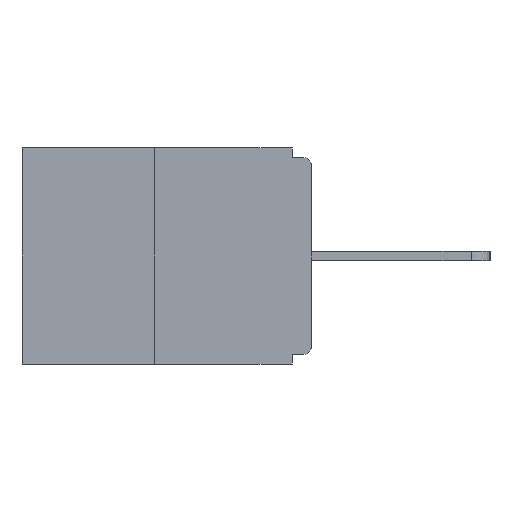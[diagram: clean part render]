
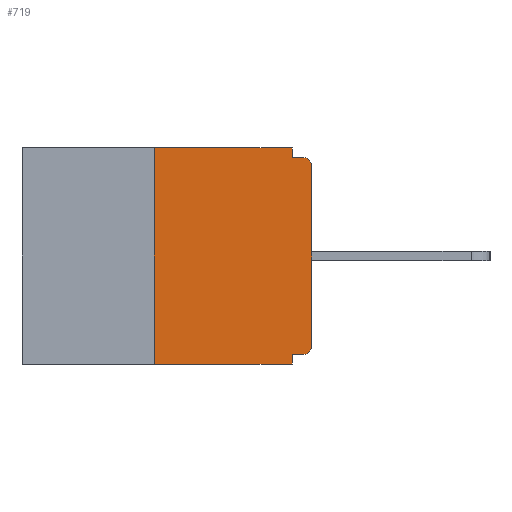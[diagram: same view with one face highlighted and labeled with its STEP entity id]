
A CAD part, left-side view. The second image highlights one B-rep face of the part: STEP entity #719.
In plain terms, the highlighted planar face has unit normal (-1, 0, 0).
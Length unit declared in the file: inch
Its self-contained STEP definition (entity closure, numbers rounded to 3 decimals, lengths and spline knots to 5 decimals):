
#126 = DIRECTION ( 'NONE',  ( 0., -1., 0. ) ) ;
#239 = DIRECTION ( 'NONE',  ( 0., 0., 1. ) ) ;
#290 = DIRECTION ( 'NONE',  ( 0., -1., 0. ) ) ;
#591 = VECTOR ( 'NONE', #10116, 39.37008 ) ;
#592 = VECTOR ( 'NONE', #1793, 39.37008 ) ;
#637 = EDGE_CURVE ( 'NONE', #10291, #11507, #8738, .T. ) ;
#719 = ADVANCED_FACE ( 'NONE', ( #7447 ), #3666, .F. ) ;
#789 = ORIENTED_EDGE ( 'NONE', *, *, #4757, .F. ) ;
#863 = LINE ( 'NONE', #10939, #592 ) ;
#873 = CARTESIAN_POINT ( 'NONE',  ( 0., 0.25, 0. ) ) ;
#1704 = CARTESIAN_POINT ( 'NONE',  ( 0., 0.46, 0. ) ) ;
#1740 = DIRECTION ( 'NONE',  ( -1., 0., 0. ) ) ;
#1793 = DIRECTION ( 'NONE',  ( 0., 0., 1. ) ) ;
#1847 = LINE ( 'NONE', #11578, #3069 ) ;
#1910 = CIRCLE ( 'NONE', #5224, 0.015 ) ;
#2091 = VERTEX_POINT ( 'NONE', #6015 ) ;
#2169 = DIRECTION ( 'NONE',  ( 0., 0., -1. ) ) ;
#2227 = DIRECTION ( 'NONE',  ( -1., 0., 0. ) ) ;
#2331 = ORIENTED_EDGE ( 'NONE', *, *, #2547, .T. ) ;
#2342 = EDGE_CURVE ( 'NONE', #5936, #8903, #7374, .T. ) ;
#2483 = ORIENTED_EDGE ( 'NONE', *, *, #2775, .T. ) ;
#2547 = EDGE_CURVE ( 'NONE', #4592, #10291, #863, .T. ) ;
#2624 = CARTESIAN_POINT ( 'NONE',  ( 0., 0.46, 0. ) ) ;
#2694 = VERTEX_POINT ( 'NONE', #5092 ) ;
#2775 = EDGE_CURVE ( 'NONE', #8818, #2091, #6390, .T. ) ;
#2864 = VECTOR ( 'NONE', #290, 39.37008 ) ;
#3030 = LINE ( 'NONE', #4143, #8489 ) ;
#3069 = VECTOR ( 'NONE', #12545, 39.37008 ) ;
#3420 = EDGE_CURVE ( 'NONE', #8818, #4256, #3030, .T. ) ;
#3666 = PLANE ( 'NONE',  #6430 ) ;
#4143 = CARTESIAN_POINT ( 'NONE',  ( 0., 0.25, 0. ) ) ;
#4256 = VERTEX_POINT ( 'NONE', #873 ) ;
#4377 = DIRECTION ( 'NONE',  ( 0., 1., 0. ) ) ;
#4575 = EDGE_CURVE ( 'NONE', #8903, #2091, #1847, .T. ) ;
#4592 = VERTEX_POINT ( 'NONE', #5552 ) ;
#4757 = EDGE_CURVE ( 'NONE', #2694, #11507, #11954, .T. ) ;
#5068 = EDGE_LOOP ( 'NONE', ( #11015, #7765, #2483, #12717, #10678, #7338, #2331, #10615, #789, #6046 ) ) ;
#5092 = CARTESIAN_POINT ( 'NONE',  ( 0., 0.031, -0.015 ) ) ;
#5144 = CARTESIAN_POINT ( 'NONE',  ( 0., 0., -0.015 ) ) ;
#5224 = AXIS2_PLACEMENT_3D ( 'NONE', #12027, #2227, #2169 ) ;
#5390 = CARTESIAN_POINT ( 'NONE',  ( 0., 0.031, 0. ) ) ;
#5540 = EDGE_CURVE ( 'NONE', #5936, #4592, #1910, .T. ) ;
#5552 = CARTESIAN_POINT ( 'NONE',  ( 0., 0., -0.313 ) ) ;
#5571 = DIRECTION ( 'NONE',  ( 0., 0., -1. ) ) ;
#5632 = DIRECTION ( 'NONE',  ( 0., 0., -1. ) ) ;
#5936 = VERTEX_POINT ( 'NONE', #6125 ) ;
#6015 = CARTESIAN_POINT ( 'NONE',  ( 0., 0.031, -0.343 ) ) ;
#6046 = ORIENTED_EDGE ( 'NONE', *, *, #6578, .F. ) ;
#6125 = CARTESIAN_POINT ( 'NONE',  ( 0., 0.015, -0.328 ) ) ;
#6169 = CARTESIAN_POINT ( 'NONE',  ( 0., 0.031, -0.328 ) ) ;
#6390 = LINE ( 'NONE', #8430, #2864 ) ;
#6430 = AXIS2_PLACEMENT_3D ( 'NONE', #2624, #10444, #5632 ) ;
#6578 = EDGE_CURVE ( 'NONE', #9125, #2694, #9363, .T. ) ;
#6613 = DIRECTION ( 'NONE',  ( 0., -1., 0. ) ) ;
#7257 = AXIS2_PLACEMENT_3D ( 'NONE', #12316, #1740, #5571 ) ;
#7297 = EDGE_CURVE ( 'NONE', #4256, #9125, #11570, .T. ) ;
#7338 = ORIENTED_EDGE ( 'NONE', *, *, #5540, .T. ) ;
#7374 = LINE ( 'NONE', #8422, #12171 ) ;
#7422 = CARTESIAN_POINT ( 'NONE',  ( 0., 0.015, -0.015 ) ) ;
#7447 = FACE_OUTER_BOUND ( 'NONE', #5068, .T. ) ;
#7634 = VECTOR ( 'NONE', #126, 39.37008 ) ;
#7658 = CARTESIAN_POINT ( 'NONE',  ( 0., 0., -0.03 ) ) ;
#7765 = ORIENTED_EDGE ( 'NONE', *, *, #3420, .F. ) ;
#8422 = CARTESIAN_POINT ( 'NONE',  ( 0., 0., -0.328 ) ) ;
#8430 = CARTESIAN_POINT ( 'NONE',  ( 0., 0.46, -0.343 ) ) ;
#8489 = VECTOR ( 'NONE', #239, 39.37008 ) ;
#8738 = CIRCLE ( 'NONE', #7257, 0.015 ) ;
#8818 = VERTEX_POINT ( 'NONE', #9181 ) ;
#8849 = CARTESIAN_POINT ( 'NONE',  ( 0., 0.031, 0. ) ) ;
#8903 = VERTEX_POINT ( 'NONE', #6169 ) ;
#9125 = VERTEX_POINT ( 'NONE', #8849 ) ;
#9181 = CARTESIAN_POINT ( 'NONE',  ( 0., 0.25, -0.343 ) ) ;
#9363 = LINE ( 'NONE', #5390, #591 ) ;
#10116 = DIRECTION ( 'NONE',  ( 0., 0., -1. ) ) ;
#10291 = VERTEX_POINT ( 'NONE', #7658 ) ;
#10444 = DIRECTION ( 'NONE',  ( 1., 0., 0. ) ) ;
#10615 = ORIENTED_EDGE ( 'NONE', *, *, #637, .T. ) ;
#10678 = ORIENTED_EDGE ( 'NONE', *, *, #2342, .F. ) ;
#10939 = CARTESIAN_POINT ( 'NONE',  ( 0., 0., 0. ) ) ;
#11015 = ORIENTED_EDGE ( 'NONE', *, *, #7297, .F. ) ;
#11507 = VERTEX_POINT ( 'NONE', #7422 ) ;
#11570 = LINE ( 'NONE', #1704, #12643 ) ;
#11578 = CARTESIAN_POINT ( 'NONE',  ( 0., 0.031, -0.343 ) ) ;
#11954 = LINE ( 'NONE', #5144, #7634 ) ;
#12027 = CARTESIAN_POINT ( 'NONE',  ( 0., 0.015, -0.313 ) ) ;
#12171 = VECTOR ( 'NONE', #4377, 39.37008 ) ;
#12316 = CARTESIAN_POINT ( 'NONE',  ( 0., 0.015, -0.03 ) ) ;
#12545 = DIRECTION ( 'NONE',  ( 0., 0., -1. ) ) ;
#12643 = VECTOR ( 'NONE', #6613, 39.37008 ) ;
#12717 = ORIENTED_EDGE ( 'NONE', *, *, #4575, .F. ) ;
